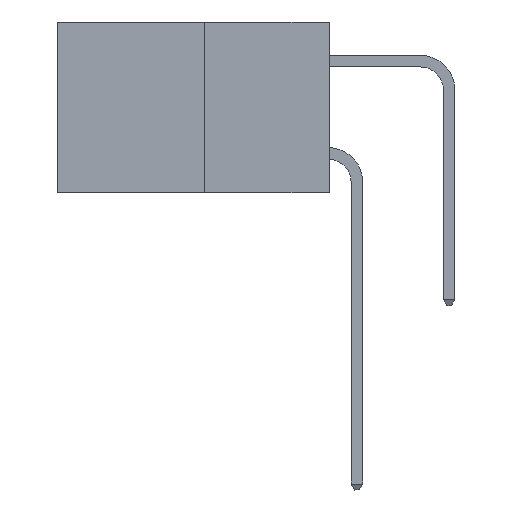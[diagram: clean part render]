
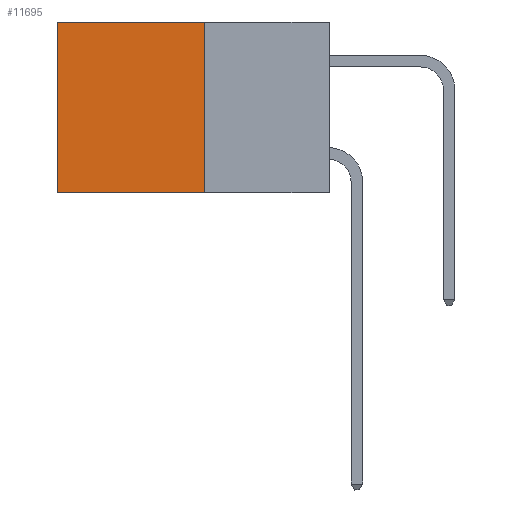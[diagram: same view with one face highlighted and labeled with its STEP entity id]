
A CAD part, left-side view. The second image highlights one B-rep face of the part: STEP entity #11695.
In plain terms, the highlighted planar face has unit normal (-1, 0, 0).
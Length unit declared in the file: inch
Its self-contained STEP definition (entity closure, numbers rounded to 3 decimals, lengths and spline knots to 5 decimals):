
#1460 = EDGE_CURVE ( 'NONE', #17411, #20105, #4287, .T. ) ;
#1505 = CARTESIAN_POINT ( 'NONE',  ( 0.277, 0.27, -0.37 ) ) ;
#2412 = CARTESIAN_POINT ( 'NONE',  ( 0.277, 0.27, 0. ) ) ;
#4287 = LINE ( 'NONE', #2412, #21468 ) ;
#4709 = CARTESIAN_POINT ( 'NONE',  ( 0.277, 0.27, -0.37 ) ) ;
#4907 = ORIENTED_EDGE ( 'NONE', *, *, #23349, .F. ) ;
#5828 = CARTESIAN_POINT ( 'NONE',  ( 0.277, 0.59, -0.37 ) ) ;
#6561 = CARTESIAN_POINT ( 'NONE',  ( 0.277, 0.59, -0.37 ) ) ;
#6863 = DIRECTION ( 'NONE',  ( 0., 1., 0. ) ) ;
#6965 = VECTOR ( 'NONE', #7163, 39.37008 ) ;
#7163 = DIRECTION ( 'NONE',  ( 0., 1., 0. ) ) ;
#8270 = VECTOR ( 'NONE', #8298, 39.37008 ) ;
#8298 = DIRECTION ( 'NONE',  ( 0., 0., -1. ) ) ;
#8381 = LINE ( 'NONE', #1505, #20597 ) ;
#9870 = EDGE_CURVE ( 'NONE', #20105, #10052, #26908, .T. ) ;
#10052 = VERTEX_POINT ( 'NONE', #6561 ) ;
#11695 = ADVANCED_FACE ( 'NONE', ( #29412 ), #26993, .F. ) ;
#12430 = CARTESIAN_POINT ( 'NONE',  ( 0.277, 0.27, -0.37 ) ) ;
#14181 = ORIENTED_EDGE ( 'NONE', *, *, #9870, .T. ) ;
#14236 = LINE ( 'NONE', #4709, #6965 ) ;
#14883 = DIRECTION ( 'NONE',  ( 0., 0., -1. ) ) ;
#16101 = DIRECTION ( 'NONE',  ( 0., 0., -1. ) ) ;
#16202 = EDGE_LOOP ( 'NONE', ( #14181, #4907, #27333, #26505 ) ) ;
#17411 = VERTEX_POINT ( 'NONE', #23856 ) ;
#20105 = VERTEX_POINT ( 'NONE', #31068 ) ;
#20450 = CARTESIAN_POINT ( 'NONE',  ( 0.277, 0.27, -0.37 ) ) ;
#20597 = VECTOR ( 'NONE', #16101, 39.37008 ) ;
#21468 = VECTOR ( 'NONE', #6863, 39.37008 ) ;
#23349 = EDGE_CURVE ( 'NONE', #31144, #10052, #14236, .T. ) ;
#23856 = CARTESIAN_POINT ( 'NONE',  ( 0.277, 0.27, 0. ) ) ;
#26505 = ORIENTED_EDGE ( 'NONE', *, *, #1460, .T. ) ;
#26908 = LINE ( 'NONE', #5828, #8270 ) ;
#26993 = PLANE ( 'NONE',  #30397 ) ;
#27333 = ORIENTED_EDGE ( 'NONE', *, *, #30633, .F. ) ;
#29412 = FACE_OUTER_BOUND ( 'NONE', #16202, .T. ) ;
#29452 = DIRECTION ( 'NONE',  ( 1., 0., 0. ) ) ;
#30397 = AXIS2_PLACEMENT_3D ( 'NONE', #12430, #29452, #14883 ) ;
#30633 = EDGE_CURVE ( 'NONE', #17411, #31144, #8381, .T. ) ;
#31068 = CARTESIAN_POINT ( 'NONE',  ( 0.277, 0.59, 0. ) ) ;
#31144 = VERTEX_POINT ( 'NONE', #20450 ) ;
